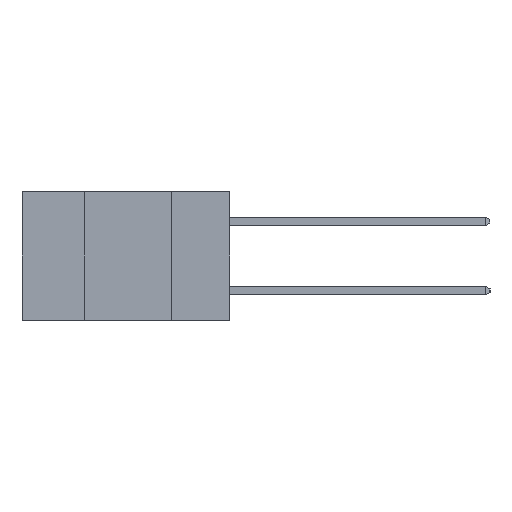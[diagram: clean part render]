
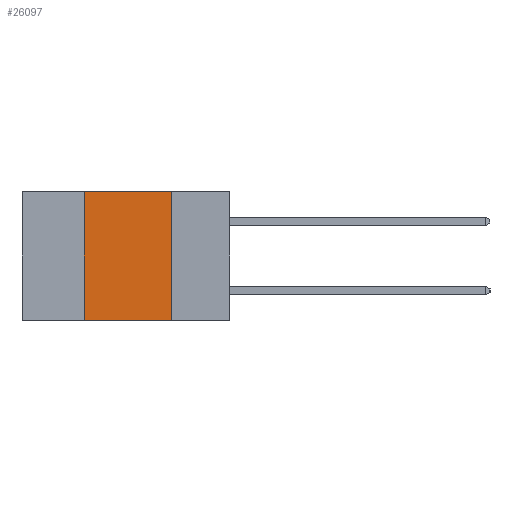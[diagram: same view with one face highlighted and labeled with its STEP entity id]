
A CAD part, left-side view. The second image highlights one B-rep face of the part: STEP entity #26097.
In plain terms, the highlighted planar face has unit normal (-1, 0, 0).
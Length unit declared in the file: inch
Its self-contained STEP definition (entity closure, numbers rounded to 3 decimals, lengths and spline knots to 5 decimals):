
#66 = EDGE_CURVE ( 'NONE', #16547, #3883, #8191, .T. ) ;
#564 = DIRECTION ( 'NONE',  ( 0., 0., -1. ) ) ;
#1942 = ORIENTED_EDGE ( 'NONE', *, *, #6363, .F. ) ;
#2693 = VECTOR ( 'NONE', #3263, 39.37008 ) ;
#2801 = DIRECTION ( 'NONE',  ( 0., 0., 1. ) ) ;
#2866 = EDGE_CURVE ( 'NONE', #3883, #4288, #8038, .T. ) ;
#3049 = EDGE_LOOP ( 'NONE', ( #14754, #8720, #1942, #17563 ) ) ;
#3263 = DIRECTION ( 'NONE',  ( 0., -1., 0. ) ) ;
#3883 = VERTEX_POINT ( 'NONE', #15584 ) ;
#4288 = VERTEX_POINT ( 'NONE', #23038 ) ;
#4450 = VERTEX_POINT ( 'NONE', #23532 ) ;
#6363 = EDGE_CURVE ( 'NONE', #4450, #16547, #6464, .T. ) ;
#6464 = LINE ( 'NONE', #20950, #20644 ) ;
#7529 = EDGE_CURVE ( 'NONE', #4450, #4288, #9577, .T. ) ;
#8038 = LINE ( 'NONE', #20926, #23397 ) ;
#8191 = LINE ( 'NONE', #19850, #2693 ) ;
#8720 = ORIENTED_EDGE ( 'NONE', *, *, #66, .F. ) ;
#8796 = PLANE ( 'NONE',  #15920 ) ;
#9577 = LINE ( 'NONE', #14473, #14346 ) ;
#12861 = DIRECTION ( 'NONE',  ( 1., 0., 0. ) ) ;
#14346 = VECTOR ( 'NONE', #16507, 39.37008 ) ;
#14473 = CARTESIAN_POINT ( 'NONE',  ( 0., 0.6, -0.37 ) ) ;
#14754 = ORIENTED_EDGE ( 'NONE', *, *, #2866, .F. ) ;
#15584 = CARTESIAN_POINT ( 'NONE',  ( 0., 0.17, 0. ) ) ;
#15920 = AXIS2_PLACEMENT_3D ( 'NONE', #22818, #12861, #564 ) ;
#16507 = DIRECTION ( 'NONE',  ( 0., -1., 0. ) ) ;
#16547 = VERTEX_POINT ( 'NONE', #19265 ) ;
#17563 = ORIENTED_EDGE ( 'NONE', *, *, #7529, .T. ) ;
#19265 = CARTESIAN_POINT ( 'NONE',  ( 0., 0.42, 0. ) ) ;
#19850 = CARTESIAN_POINT ( 'NONE',  ( 0., 0.6, 0. ) ) ;
#20644 = VECTOR ( 'NONE', #2801, 39.37008 ) ;
#20926 = CARTESIAN_POINT ( 'NONE',  ( 0., 0.17, -0.37 ) ) ;
#20950 = CARTESIAN_POINT ( 'NONE',  ( 0., 0.42, -0.37 ) ) ;
#21628 = FACE_OUTER_BOUND ( 'NONE', #3049, .T. ) ;
#21848 = DIRECTION ( 'NONE',  ( 0., 0., -1. ) ) ;
#22818 = CARTESIAN_POINT ( 'NONE',  ( 0., 0.6, 0. ) ) ;
#23038 = CARTESIAN_POINT ( 'NONE',  ( 0., 0.17, -0.37 ) ) ;
#23397 = VECTOR ( 'NONE', #21848, 39.37008 ) ;
#23532 = CARTESIAN_POINT ( 'NONE',  ( 0., 0.42, -0.37 ) ) ;
#26097 = ADVANCED_FACE ( 'NONE', ( #21628 ), #8796, .F. ) ;
